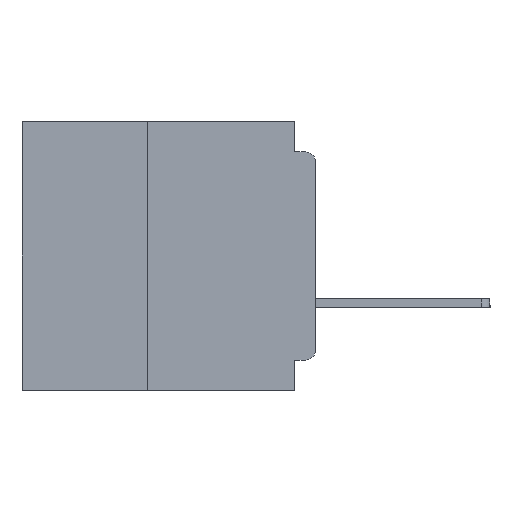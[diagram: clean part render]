
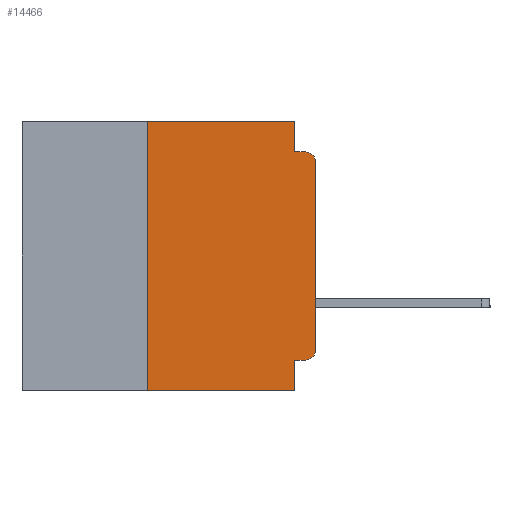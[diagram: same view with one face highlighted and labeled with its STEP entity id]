
A CAD part, left-side view. The second image highlights one B-rep face of the part: STEP entity #14466.
In plain terms, the highlighted planar face has unit normal (-1, 0, 0).
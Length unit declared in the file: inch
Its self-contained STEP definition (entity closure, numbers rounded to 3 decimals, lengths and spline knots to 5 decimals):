
#759 = CARTESIAN_POINT ( 'NONE',  ( 0., 0., 0. ) ) ;
#1154 = VECTOR ( 'NONE', #14118, 39.37008 ) ;
#1441 = VECTOR ( 'NONE', #26143, 39.37008 ) ;
#1753 = CARTESIAN_POINT ( 'NONE',  ( 0., 0.437, 0. ) ) ;
#1890 = ORIENTED_EDGE ( 'NONE', *, *, #11196, .F. ) ;
#2995 = VERTEX_POINT ( 'NONE', #30563 ) ;
#3358 = EDGE_CURVE ( 'NONE', #34644, #2995, #21877, .T. ) ;
#3415 = VERTEX_POINT ( 'NONE', #14296 ) ;
#3452 = VERTEX_POINT ( 'NONE', #29606 ) ;
#3561 = ORIENTED_EDGE ( 'NONE', *, *, #6124, .T. ) ;
#4061 = AXIS2_PLACEMENT_3D ( 'NONE', #34874, #16705, #37824 ) ;
#4266 = CARTESIAN_POINT ( 'NONE',  ( 0., 0.031, 0. ) ) ;
#4533 = VECTOR ( 'NONE', #19758, 39.37008 ) ;
#4781 = DIRECTION ( 'NONE',  ( 1., 0., 0. ) ) ;
#5257 = ORIENTED_EDGE ( 'NONE', *, *, #21386, .F. ) ;
#5673 = VERTEX_POINT ( 'NONE', #11452 ) ;
#5806 = AXIS2_PLACEMENT_3D ( 'NONE', #1753, #4781, #26063 ) ;
#6124 = EDGE_CURVE ( 'NONE', #5673, #35769, #31136, .T. ) ;
#7280 = DIRECTION ( 'NONE',  ( 0., 0., -1. ) ) ;
#8978 = LINE ( 'NONE', #11276, #15828 ) ;
#9855 = DIRECTION ( 'NONE',  ( -1., 0., 0. ) ) ;
#10645 = AXIS2_PLACEMENT_3D ( 'NONE', #28068, #9855, #31123 ) ;
#11196 = EDGE_CURVE ( 'NONE', #37056, #3452, #8978, .T. ) ;
#11276 = CARTESIAN_POINT ( 'NONE',  ( 0., 0.031, -0.4 ) ) ;
#11452 = CARTESIAN_POINT ( 'NONE',  ( 0., 0.015, -0.355 ) ) ;
#12261 = VERTEX_POINT ( 'NONE', #33415 ) ;
#12616 = LINE ( 'NONE', #31997, #4533 ) ;
#13223 = EDGE_CURVE ( 'NONE', #19327, #3452, #12616, .T. ) ;
#13279 = VECTOR ( 'NONE', #25060, 39.37008 ) ;
#14052 = LINE ( 'NONE', #21385, #29288 ) ;
#14118 = DIRECTION ( 'NONE',  ( 0., 0., 1. ) ) ;
#14127 = ORIENTED_EDGE ( 'NONE', *, *, #3358, .F. ) ;
#14269 = EDGE_CURVE ( 'NONE', #12261, #2995, #35827, .T. ) ;
#14296 = CARTESIAN_POINT ( 'NONE',  ( 0., 0.031, 0. ) ) ;
#14466 = ADVANCED_FACE ( 'NONE', ( #38087 ), #37970, .F. ) ;
#14553 = VECTOR ( 'NONE', #20709, 39.37008 ) ;
#15114 = VECTOR ( 'NONE', #7280, 39.37008 ) ;
#15551 = EDGE_CURVE ( 'NONE', #35769, #12261, #37394, .T. ) ;
#15828 = VECTOR ( 'NONE', #29497, 39.37008 ) ;
#16705 = DIRECTION ( 'NONE',  ( -1., 0., 0. ) ) ;
#18264 = LINE ( 'NONE', #32344, #1154 ) ;
#18371 = EDGE_CURVE ( 'NONE', #5673, #37056, #14052, .T. ) ;
#19327 = VERTEX_POINT ( 'NONE', #35187 ) ;
#19346 = EDGE_CURVE ( 'NONE', #19327, #19508, #18264, .T. ) ;
#19508 = VERTEX_POINT ( 'NONE', #24119 ) ;
#19758 = DIRECTION ( 'NONE',  ( 0., -1., 0. ) ) ;
#20709 = DIRECTION ( 'NONE',  ( 0., -1., 0. ) ) ;
#20770 = ORIENTED_EDGE ( 'NONE', *, *, #13223, .T. ) ;
#21018 = ORIENTED_EDGE ( 'NONE', *, *, #14269, .T. ) ;
#21295 = ORIENTED_EDGE ( 'NONE', *, *, #18371, .F. ) ;
#21385 = CARTESIAN_POINT ( 'NONE',  ( 0., 0., -0.355 ) ) ;
#21386 = EDGE_CURVE ( 'NONE', #3415, #34644, #39170, .T. ) ;
#21877 = LINE ( 'NONE', #35235, #1441 ) ;
#22652 = LINE ( 'NONE', #32838, #14553 ) ;
#23210 = EDGE_LOOP ( 'NONE', ( #29281, #21018, #14127, #5257, #23282, #24748, #20770, #1890, #21295, #3561 ) ) ;
#23282 = ORIENTED_EDGE ( 'NONE', *, *, #27497, .F. ) ;
#24119 = CARTESIAN_POINT ( 'NONE',  ( 0., 0.25, 0. ) ) ;
#24748 = ORIENTED_EDGE ( 'NONE', *, *, #19346, .F. ) ;
#25060 = DIRECTION ( 'NONE',  ( 0., 0., 1. ) ) ;
#25954 = CARTESIAN_POINT ( 'NONE',  ( 0., 0.031, -0.045 ) ) ;
#26063 = DIRECTION ( 'NONE',  ( 0., 0., -1. ) ) ;
#26143 = DIRECTION ( 'NONE',  ( 0., -1., 0. ) ) ;
#27497 = EDGE_CURVE ( 'NONE', #19508, #3415, #22652, .T. ) ;
#28068 = CARTESIAN_POINT ( 'NONE',  ( 0., 0.015, -0.06 ) ) ;
#29281 = ORIENTED_EDGE ( 'NONE', *, *, #15551, .T. ) ;
#29288 = VECTOR ( 'NONE', #36448, 39.37008 ) ;
#29497 = DIRECTION ( 'NONE',  ( 0., 0., -1. ) ) ;
#29606 = CARTESIAN_POINT ( 'NONE',  ( 0., 0.031, -0.4 ) ) ;
#30563 = CARTESIAN_POINT ( 'NONE',  ( 0., 0.015, -0.045 ) ) ;
#31123 = DIRECTION ( 'NONE',  ( 0., 0., -1. ) ) ;
#31136 = CIRCLE ( 'NONE', #4061, 0.015 ) ;
#31706 = CARTESIAN_POINT ( 'NONE',  ( 0., 0., -0.34 ) ) ;
#31997 = CARTESIAN_POINT ( 'NONE',  ( 0., 0.437, -0.4 ) ) ;
#32344 = CARTESIAN_POINT ( 'NONE',  ( 0., 0.25, -0.4 ) ) ;
#32838 = CARTESIAN_POINT ( 'NONE',  ( 0., 0.437, 0. ) ) ;
#33415 = CARTESIAN_POINT ( 'NONE',  ( 0., 0., -0.06 ) ) ;
#34644 = VERTEX_POINT ( 'NONE', #25954 ) ;
#34874 = CARTESIAN_POINT ( 'NONE',  ( 0., 0.015, -0.34 ) ) ;
#35187 = CARTESIAN_POINT ( 'NONE',  ( 0., 0.25, -0.4 ) ) ;
#35235 = CARTESIAN_POINT ( 'NONE',  ( 0., 0., -0.045 ) ) ;
#35769 = VERTEX_POINT ( 'NONE', #31706 ) ;
#35827 = CIRCLE ( 'NONE', #10645, 0.015 ) ;
#36448 = DIRECTION ( 'NONE',  ( 0., 1., 0. ) ) ;
#37056 = VERTEX_POINT ( 'NONE', #39030 ) ;
#37394 = LINE ( 'NONE', #759, #13279 ) ;
#37824 = DIRECTION ( 'NONE',  ( 0., 0., -1. ) ) ;
#37970 = PLANE ( 'NONE',  #5806 ) ;
#38087 = FACE_OUTER_BOUND ( 'NONE', #23210, .T. ) ;
#39030 = CARTESIAN_POINT ( 'NONE',  ( 0., 0.031, -0.355 ) ) ;
#39170 = LINE ( 'NONE', #4266, #15114 ) ;
